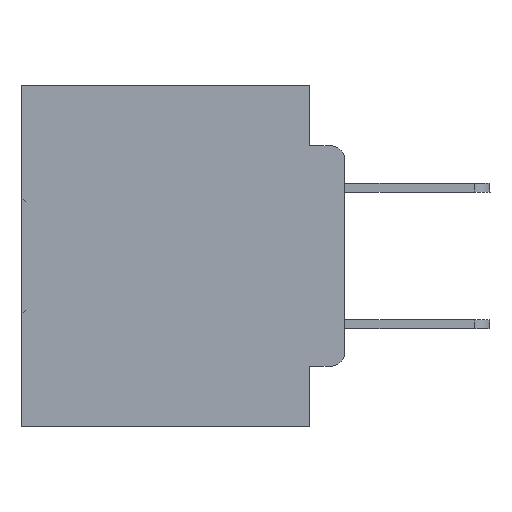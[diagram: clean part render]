
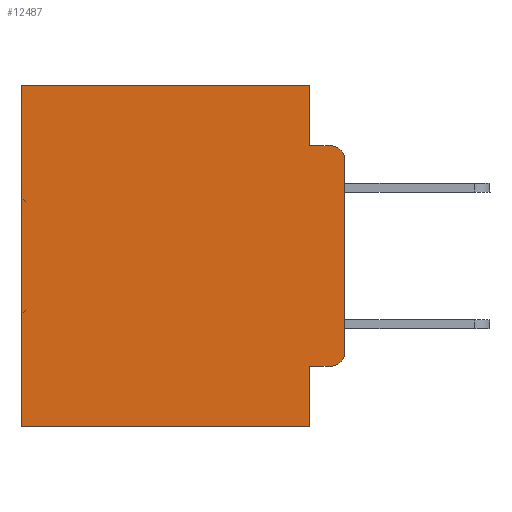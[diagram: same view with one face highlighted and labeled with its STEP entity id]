
A CAD part, left-side view. The second image highlights one B-rep face of the part: STEP entity #12487.
In plain terms, the highlighted planar face has unit normal (-1, 0, 0).
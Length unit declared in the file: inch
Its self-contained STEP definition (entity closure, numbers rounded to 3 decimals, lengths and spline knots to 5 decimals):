
#321 = CARTESIAN_POINT ( 'NONE',  ( 0.298, 0.051, -0.4115 ) ) ;
#795 = VERTEX_POINT ( 'NONE', #22747 ) ;
#1311 = ORIENTED_EDGE ( 'NONE', *, *, #13584, .F. ) ;
#1325 = CARTESIAN_POINT ( 'NONE',  ( 0.298, 0., -0.1085 ) ) ;
#1774 = EDGE_CURVE ( 'NONE', #32672, #23924, #17986, .T. ) ;
#2185 = VECTOR ( 'NONE', #2300, 39.37008 ) ;
#2208 = VECTOR ( 'NONE', #6778, 39.37008 ) ;
#2300 = DIRECTION ( 'NONE',  ( 0., 0., -1. ) ) ;
#2309 = AXIS2_PLACEMENT_3D ( 'NONE', #18599, #21226, #28790 ) ;
#3894 = VERTEX_POINT ( 'NONE', #31300 ) ;
#4041 = CARTESIAN_POINT ( 'NONE',  ( 0.298, 0., -0.5 ) ) ;
#5169 = VECTOR ( 'NONE', #15189, 39.37008 ) ;
#5362 = EDGE_CURVE ( 'NONE', #14059, #24031, #27702, .T. ) ;
#5633 = CARTESIAN_POINT ( 'NONE',  ( 0.298, 0., 0. ) ) ;
#6778 = DIRECTION ( 'NONE',  ( 0., -1., 0. ) ) ;
#7085 = EDGE_CURVE ( 'NONE', #24031, #29842, #31767, .T. ) ;
#7170 = CARTESIAN_POINT ( 'NONE',  ( 0.298, 0.02, -0.0885 ) ) ;
#8120 = EDGE_CURVE ( 'NONE', #25571, #795, #23446, .T. ) ;
#9504 = CIRCLE ( 'NONE', #16717, 0.02 ) ;
#10168 = EDGE_LOOP ( 'NONE', ( #30464, #28845, #16191, #27690, #16991, #31487, #27805, #1311, #28524, #20747 ) ) ;
#10514 = EDGE_CURVE ( 'NONE', #14059, #3894, #27003, .T. ) ;
#10575 = CARTESIAN_POINT ( 'NONE',  ( 0.298, 0.02, -0.1085 ) ) ;
#11144 = CARTESIAN_POINT ( 'NONE',  ( 0.298, 0.051, -0.0885 ) ) ;
#11300 = FACE_OUTER_BOUND ( 'NONE', #10168, .T. ) ;
#11362 = LINE ( 'NONE', #321, #26116 ) ;
#11443 = EDGE_CURVE ( 'NONE', #32629, #31148, #11362, .T. ) ;
#11543 = DIRECTION ( 'NONE',  ( -1., 0., 0. ) ) ;
#12487 = ADVANCED_FACE ( 'NONE', ( #11300 ), #28684, .F. ) ;
#12595 = DIRECTION ( 'NONE',  ( 0., 0., -1. ) ) ;
#13310 = DIRECTION ( 'NONE',  ( 0., -1., 0. ) ) ;
#13442 = DIRECTION ( 'NONE',  ( -1., 0., 0. ) ) ;
#13580 = CARTESIAN_POINT ( 'NONE',  ( 0.298, 0.473, -0.5 ) ) ;
#13584 = EDGE_CURVE ( 'NONE', #32629, #32672, #15761, .T. ) ;
#13677 = CARTESIAN_POINT ( 'NONE',  ( 0.298, 0.051, -0.5 ) ) ;
#14059 = VERTEX_POINT ( 'NONE', #26214 ) ;
#14069 = AXIS2_PLACEMENT_3D ( 'NONE', #10575, #13442, #31880 ) ;
#14363 = EDGE_CURVE ( 'NONE', #31148, #795, #9504, .T. ) ;
#14966 = CARTESIAN_POINT ( 'NONE',  ( 0.298, 0.051, 0. ) ) ;
#15189 = DIRECTION ( 'NONE',  ( 0., 0., -1. ) ) ;
#15451 = EDGE_CURVE ( 'NONE', #25571, #29842, #28413, .T. ) ;
#15761 = LINE ( 'NONE', #15832, #2185 ) ;
#15832 = CARTESIAN_POINT ( 'NONE',  ( 0.298, 0.051, 0. ) ) ;
#16191 = ORIENTED_EDGE ( 'NONE', *, *, #7085, .F. ) ;
#16482 = VECTOR ( 'NONE', #26367, 39.37008 ) ;
#16717 = AXIS2_PLACEMENT_3D ( 'NONE', #27566, #11543, #30208 ) ;
#16991 = ORIENTED_EDGE ( 'NONE', *, *, #10514, .T. ) ;
#17986 = LINE ( 'NONE', #4041, #27410 ) ;
#17996 = VECTOR ( 'NONE', #27880, 39.37008 ) ;
#18543 = CARTESIAN_POINT ( 'NONE',  ( 0.298, 0.02, -0.4115 ) ) ;
#18599 = CARTESIAN_POINT ( 'NONE',  ( 0.298, 0., 0. ) ) ;
#20747 = ORIENTED_EDGE ( 'NONE', *, *, #14363, .T. ) ;
#21226 = DIRECTION ( 'NONE',  ( 1., 0., 0. ) ) ;
#22747 = CARTESIAN_POINT ( 'NONE',  ( 0.298, 0., -0.3915 ) ) ;
#23446 = LINE ( 'NONE', #5633, #16482 ) ;
#23924 = VERTEX_POINT ( 'NONE', #13580 ) ;
#24031 = VERTEX_POINT ( 'NONE', #11144 ) ;
#24192 = CARTESIAN_POINT ( 'NONE',  ( 0.298, 0.051, -0.4115 ) ) ;
#24943 = EDGE_CURVE ( 'NONE', #3894, #23924, #32568, .T. ) ;
#25571 = VERTEX_POINT ( 'NONE', #1325 ) ;
#26116 = VECTOR ( 'NONE', #13310, 39.37008 ) ;
#26214 = CARTESIAN_POINT ( 'NONE',  ( 0.298, 0.051, 0. ) ) ;
#26367 = DIRECTION ( 'NONE',  ( 0., 0., -1. ) ) ;
#27003 = LINE ( 'NONE', #27771, #17996 ) ;
#27410 = VECTOR ( 'NONE', #32614, 39.37008 ) ;
#27566 = CARTESIAN_POINT ( 'NONE',  ( 0.298, 0.02, -0.3915 ) ) ;
#27617 = CARTESIAN_POINT ( 'NONE',  ( 0.298, 0.051, -0.0885 ) ) ;
#27690 = ORIENTED_EDGE ( 'NONE', *, *, #5362, .F. ) ;
#27702 = LINE ( 'NONE', #14966, #5169 ) ;
#27771 = CARTESIAN_POINT ( 'NONE',  ( 0.298, 0., 0. ) ) ;
#27805 = ORIENTED_EDGE ( 'NONE', *, *, #1774, .F. ) ;
#27880 = DIRECTION ( 'NONE',  ( 0., 1., 0. ) ) ;
#28381 = CARTESIAN_POINT ( 'NONE',  ( 0.298, 0.473, 0. ) ) ;
#28413 = CIRCLE ( 'NONE', #14069, 0.02 ) ;
#28524 = ORIENTED_EDGE ( 'NONE', *, *, #11443, .T. ) ;
#28684 = PLANE ( 'NONE',  #2309 ) ;
#28790 = DIRECTION ( 'NONE',  ( 0., 0., -1. ) ) ;
#28845 = ORIENTED_EDGE ( 'NONE', *, *, #15451, .T. ) ;
#29842 = VERTEX_POINT ( 'NONE', #7170 ) ;
#30208 = DIRECTION ( 'NONE',  ( 0., 0., -1. ) ) ;
#30464 = ORIENTED_EDGE ( 'NONE', *, *, #8120, .F. ) ;
#31148 = VERTEX_POINT ( 'NONE', #18543 ) ;
#31300 = CARTESIAN_POINT ( 'NONE',  ( 0.298, 0.473, 0. ) ) ;
#31487 = ORIENTED_EDGE ( 'NONE', *, *, #24943, .T. ) ;
#31755 = VECTOR ( 'NONE', #12595, 39.37008 ) ;
#31767 = LINE ( 'NONE', #27617, #2208 ) ;
#31880 = DIRECTION ( 'NONE',  ( 0., 0., -1. ) ) ;
#32568 = LINE ( 'NONE', #28381, #31755 ) ;
#32614 = DIRECTION ( 'NONE',  ( 0., 1., 0. ) ) ;
#32629 = VERTEX_POINT ( 'NONE', #24192 ) ;
#32672 = VERTEX_POINT ( 'NONE', #13677 ) ;
